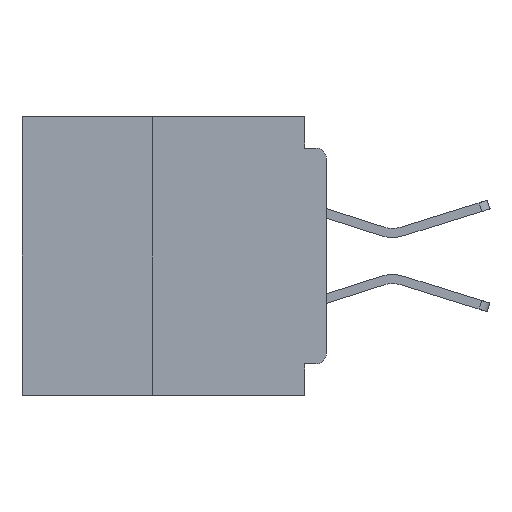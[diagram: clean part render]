
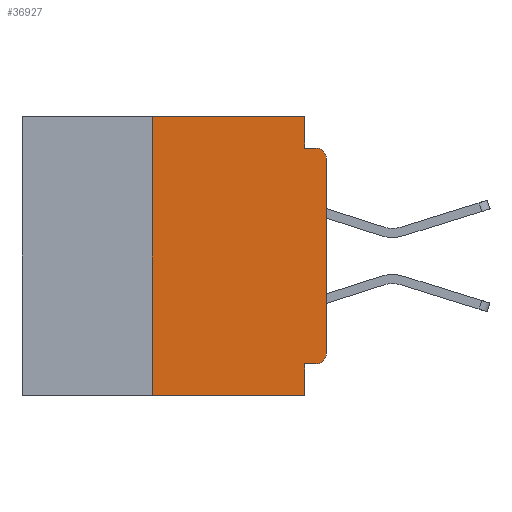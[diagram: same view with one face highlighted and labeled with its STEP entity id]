
A CAD part, left-side view. The second image highlights one B-rep face of the part: STEP entity #36927.
In plain terms, the highlighted planar face has unit normal (-1, 0, 0).
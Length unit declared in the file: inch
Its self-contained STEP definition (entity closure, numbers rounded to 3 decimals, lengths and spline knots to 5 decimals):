
#609 = ORIENTED_EDGE ( 'NONE', *, *, #35512, .F. ) ;
#1280 = VERTEX_POINT ( 'NONE', #8575 ) ;
#1448 = ORIENTED_EDGE ( 'NONE', *, *, #26084, .T. ) ;
#2780 = DIRECTION ( 'NONE',  ( 0., -1., 0. ) ) ;
#2852 = EDGE_CURVE ( 'NONE', #18992, #21174, #36394, .T. ) ;
#3528 = LINE ( 'NONE', #15346, #19283 ) ;
#3675 = EDGE_CURVE ( 'NONE', #17951, #29703, #28184, .T. ) ;
#3684 = DIRECTION ( 'NONE',  ( 0., 0., -1. ) ) ;
#3778 = VERTEX_POINT ( 'NONE', #23080 ) ;
#4747 = EDGE_CURVE ( 'NONE', #27601, #1280, #3528, .T. ) ;
#4850 = CARTESIAN_POINT ( 'NONE',  ( 0., 0.031, -0.355 ) ) ;
#4896 = VECTOR ( 'NONE', #5991, 39.37008 ) ;
#5778 = AXIS2_PLACEMENT_3D ( 'NONE', #32638, #13984, #35703 ) ;
#5854 = ORIENTED_EDGE ( 'NONE', *, *, #16494, .F. ) ;
#5991 = DIRECTION ( 'NONE',  ( 0., 0., -1. ) ) ;
#8575 = CARTESIAN_POINT ( 'NONE',  ( 0., 0.25, 0. ) ) ;
#9262 = ORIENTED_EDGE ( 'NONE', *, *, #13282, .T. ) ;
#9976 = CARTESIAN_POINT ( 'NONE',  ( 0., 0.015, -0.355 ) ) ;
#9987 = DIRECTION ( 'NONE',  ( 0., 0., 1. ) ) ;
#10527 = VECTOR ( 'NONE', #22534, 39.37008 ) ;
#11087 = CIRCLE ( 'NONE', #35793, 0.015 ) ;
#11305 = CARTESIAN_POINT ( 'NONE',  ( 0., 0.25, -0.4 ) ) ;
#11987 = VECTOR ( 'NONE', #2780, 39.37008 ) ;
#13123 = CARTESIAN_POINT ( 'NONE',  ( 0., 0., 0. ) ) ;
#13282 = EDGE_CURVE ( 'NONE', #27601, #17414, #24922, .T. ) ;
#13984 = DIRECTION ( 'NONE',  ( -1., 0., 0. ) ) ;
#14862 = ORIENTED_EDGE ( 'NONE', *, *, #30860, .T. ) ;
#15274 = CARTESIAN_POINT ( 'NONE',  ( 0., 0.437, -0.4 ) ) ;
#15346 = CARTESIAN_POINT ( 'NONE',  ( 0., 0.25, -0.4 ) ) ;
#15864 = CARTESIAN_POINT ( 'NONE',  ( 0., 0.031, 0. ) ) ;
#16042 = LINE ( 'NONE', #18132, #38753 ) ;
#16232 = EDGE_CURVE ( 'NONE', #1280, #25949, #24865, .T. ) ;
#16494 = EDGE_CURVE ( 'NONE', #29703, #17414, #16042, .T. ) ;
#16528 = DIRECTION ( 'NONE',  ( -1., 0., 0. ) ) ;
#16590 = VECTOR ( 'NONE', #37078, 39.37008 ) ;
#16890 = DIRECTION ( 'NONE',  ( 0., -1., 0. ) ) ;
#17414 = VERTEX_POINT ( 'NONE', #25441 ) ;
#17910 = EDGE_CURVE ( 'NONE', #3778, #34553, #28658, .T. ) ;
#17951 = VERTEX_POINT ( 'NONE', #9976 ) ;
#18132 = CARTESIAN_POINT ( 'NONE',  ( 0., 0.031, -0.4 ) ) ;
#18978 = EDGE_LOOP ( 'NONE', ( #28826, #14862, #22698, #609, #39104, #19436, #9262, #5854, #25126, #1448 ) ) ;
#18992 = VERTEX_POINT ( 'NONE', #27567 ) ;
#19283 = VECTOR ( 'NONE', #27827, 39.37008 ) ;
#19382 = CARTESIAN_POINT ( 'NONE',  ( 0., 0.437, 0. ) ) ;
#19418 = CARTESIAN_POINT ( 'NONE',  ( 0., 0., -0.355 ) ) ;
#19436 = ORIENTED_EDGE ( 'NONE', *, *, #4747, .F. ) ;
#21174 = VERTEX_POINT ( 'NONE', #23844 ) ;
#22492 = DIRECTION ( 'NONE',  ( 1., 0., 0. ) ) ;
#22534 = DIRECTION ( 'NONE',  ( 0., 1., 0. ) ) ;
#22698 = ORIENTED_EDGE ( 'NONE', *, *, #17910, .F. ) ;
#23080 = CARTESIAN_POINT ( 'NONE',  ( 0., 0.031, -0.045 ) ) ;
#23844 = CARTESIAN_POINT ( 'NONE',  ( 0., 0., -0.06 ) ) ;
#24865 = LINE ( 'NONE', #38513, #33081 ) ;
#24922 = LINE ( 'NONE', #15274, #16590 ) ;
#25126 = ORIENTED_EDGE ( 'NONE', *, *, #3675, .F. ) ;
#25441 = CARTESIAN_POINT ( 'NONE',  ( 0., 0.031, -0.4 ) ) ;
#25949 = VERTEX_POINT ( 'NONE', #15864 ) ;
#26084 = EDGE_CURVE ( 'NONE', #17951, #18992, #11087, .T. ) ;
#27314 = VECTOR ( 'NONE', #9987, 39.37008 ) ;
#27567 = CARTESIAN_POINT ( 'NONE',  ( 0., 0., -0.34 ) ) ;
#27601 = VERTEX_POINT ( 'NONE', #11305 ) ;
#27827 = DIRECTION ( 'NONE',  ( 0., 0., 1. ) ) ;
#28184 = LINE ( 'NONE', #19418, #10527 ) ;
#28658 = LINE ( 'NONE', #37102, #11987 ) ;
#28826 = ORIENTED_EDGE ( 'NONE', *, *, #2852, .T. ) ;
#29703 = VERTEX_POINT ( 'NONE', #4850 ) ;
#29900 = LINE ( 'NONE', #37014, #4896 ) ;
#30860 = EDGE_CURVE ( 'NONE', #21174, #34553, #30872, .T. ) ;
#30872 = CIRCLE ( 'NONE', #5778, 0.015 ) ;
#32169 = FACE_OUTER_BOUND ( 'NONE', #18978, .T. ) ;
#32638 = CARTESIAN_POINT ( 'NONE',  ( 0., 0.015, -0.06 ) ) ;
#33081 = VECTOR ( 'NONE', #16890, 39.37008 ) ;
#34553 = VERTEX_POINT ( 'NONE', #38292 ) ;
#35109 = CARTESIAN_POINT ( 'NONE',  ( 0., 0.015, -0.34 ) ) ;
#35512 = EDGE_CURVE ( 'NONE', #25949, #3778, #29900, .T. ) ;
#35703 = DIRECTION ( 'NONE',  ( 0., 0., -1. ) ) ;
#35793 = AXIS2_PLACEMENT_3D ( 'NONE', #35109, #16528, #38164 ) ;
#36394 = LINE ( 'NONE', #13123, #27314 ) ;
#36634 = DIRECTION ( 'NONE',  ( 0., 0., -1. ) ) ;
#36927 = ADVANCED_FACE ( 'NONE', ( #32169 ), #37843, .F. ) ;
#37014 = CARTESIAN_POINT ( 'NONE',  ( 0., 0.031, 0. ) ) ;
#37078 = DIRECTION ( 'NONE',  ( 0., -1., 0. ) ) ;
#37102 = CARTESIAN_POINT ( 'NONE',  ( 0., 0., -0.045 ) ) ;
#37843 = PLANE ( 'NONE',  #38237 ) ;
#38164 = DIRECTION ( 'NONE',  ( 0., 0., -1. ) ) ;
#38237 = AXIS2_PLACEMENT_3D ( 'NONE', #19382, #22492, #3684 ) ;
#38292 = CARTESIAN_POINT ( 'NONE',  ( 0., 0.015, -0.045 ) ) ;
#38513 = CARTESIAN_POINT ( 'NONE',  ( 0., 0.437, 0. ) ) ;
#38753 = VECTOR ( 'NONE', #36634, 39.37008 ) ;
#39104 = ORIENTED_EDGE ( 'NONE', *, *, #16232, .F. ) ;
